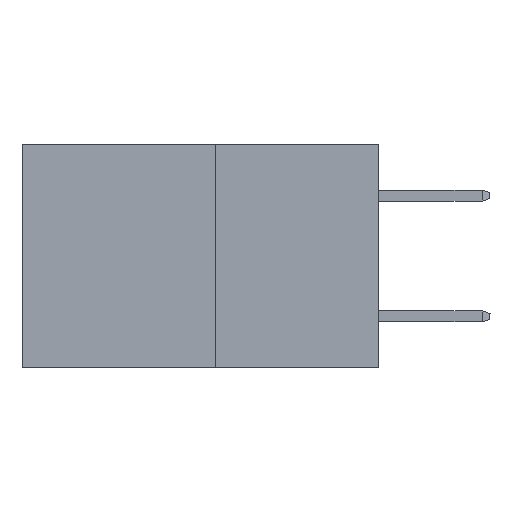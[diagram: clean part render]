
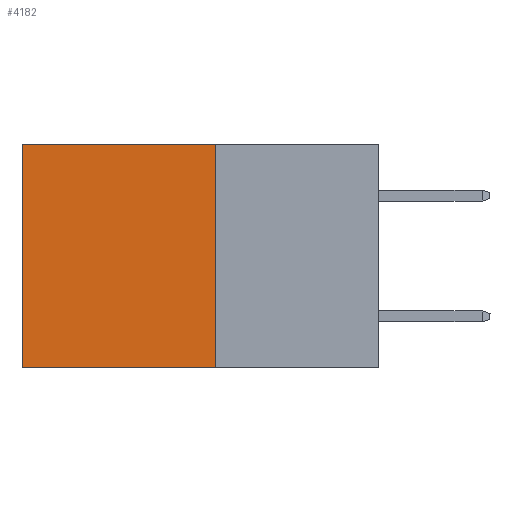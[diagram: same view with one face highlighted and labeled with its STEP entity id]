
A CAD part, left-side view. The second image highlights one B-rep face of the part: STEP entity #4182.
In plain terms, the highlighted planar face has unit normal (-1, 0, 0).
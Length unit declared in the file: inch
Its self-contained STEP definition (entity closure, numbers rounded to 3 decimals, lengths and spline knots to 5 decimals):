
#180 = LINE ( 'NONE', #13689, #19308 ) ;
#203 = DIRECTION ( 'NONE',  ( 0., 0., -1. ) ) ;
#266 = LINE ( 'NONE', #23031, #14510 ) ;
#272 = CARTESIAN_POINT ( 'NONE',  ( 0.277, 0.59, -0.37 ) ) ;
#945 = VECTOR ( 'NONE', #5550, 39.37008 ) ;
#1318 = CARTESIAN_POINT ( 'NONE',  ( 0.277, 0.59, 0. ) ) ;
#1416 = LINE ( 'NONE', #9906, #6379 ) ;
#2787 = EDGE_CURVE ( 'NONE', #14901, #16111, #15163, .T. ) ;
#4182 = ADVANCED_FACE ( 'NONE', ( #18268 ), #18753, .F. ) ;
#5550 = DIRECTION ( 'NONE',  ( 0., 1., 0. ) ) ;
#6215 = ORIENTED_EDGE ( 'NONE', *, *, #13882, .T. ) ;
#6379 = VECTOR ( 'NONE', #8207, 39.37008 ) ;
#7513 = AXIS2_PLACEMENT_3D ( 'NONE', #16893, #11469, #203 ) ;
#8207 = DIRECTION ( 'NONE',  ( 0., 0., -1. ) ) ;
#8832 = CARTESIAN_POINT ( 'NONE',  ( 0.277, 0.27, -0.37 ) ) ;
#9039 = EDGE_CURVE ( 'NONE', #12288, #14901, #1416, .T. ) ;
#9906 = CARTESIAN_POINT ( 'NONE',  ( 0.277, 0.27, -0.37 ) ) ;
#11469 = DIRECTION ( 'NONE',  ( 1., 0., 0. ) ) ;
#12288 = VERTEX_POINT ( 'NONE', #12554 ) ;
#12554 = CARTESIAN_POINT ( 'NONE',  ( 0.277, 0.27, 0. ) ) ;
#13689 = CARTESIAN_POINT ( 'NONE',  ( 0.277, 0.59, -0.37 ) ) ;
#13882 = EDGE_CURVE ( 'NONE', #21589, #16111, #180, .T. ) ;
#13894 = DIRECTION ( 'NONE',  ( 0., 1., 0. ) ) ;
#14510 = VECTOR ( 'NONE', #13894, 39.37008 ) ;
#14601 = CARTESIAN_POINT ( 'NONE',  ( 0.277, 0.27, -0.37 ) ) ;
#14901 = VERTEX_POINT ( 'NONE', #8832 ) ;
#15163 = LINE ( 'NONE', #14601, #945 ) ;
#16111 = VERTEX_POINT ( 'NONE', #272 ) ;
#16646 = ORIENTED_EDGE ( 'NONE', *, *, #2787, .F. ) ;
#16893 = CARTESIAN_POINT ( 'NONE',  ( 0.277, 0.27, -0.37 ) ) ;
#17375 = DIRECTION ( 'NONE',  ( 0., 0., -1. ) ) ;
#18268 = FACE_OUTER_BOUND ( 'NONE', #18354, .T. ) ;
#18354 = EDGE_LOOP ( 'NONE', ( #6215, #16646, #23544, #18407 ) ) ;
#18407 = ORIENTED_EDGE ( 'NONE', *, *, #22498, .T. ) ;
#18753 = PLANE ( 'NONE',  #7513 ) ;
#19308 = VECTOR ( 'NONE', #17375, 39.37008 ) ;
#21589 = VERTEX_POINT ( 'NONE', #1318 ) ;
#22498 = EDGE_CURVE ( 'NONE', #12288, #21589, #266, .T. ) ;
#23031 = CARTESIAN_POINT ( 'NONE',  ( 0.277, 0.27, 0. ) ) ;
#23544 = ORIENTED_EDGE ( 'NONE', *, *, #9039, .F. ) ;
